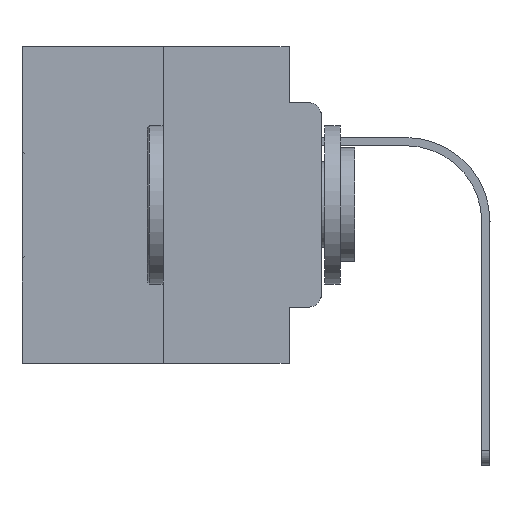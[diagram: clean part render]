
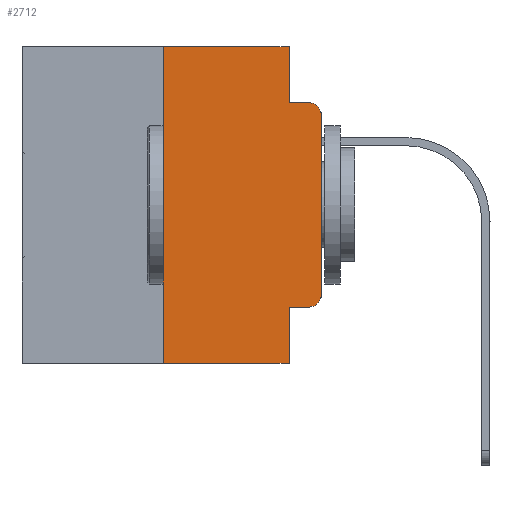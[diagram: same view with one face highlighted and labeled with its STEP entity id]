
A CAD part, left-side view. The second image highlights one B-rep face of the part: STEP entity #2712.
In plain terms, the highlighted planar face has unit normal (-1, 0, 0).
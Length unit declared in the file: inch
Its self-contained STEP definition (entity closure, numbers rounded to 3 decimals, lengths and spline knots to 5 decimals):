
#999 = EDGE_CURVE ( 'NONE', #12765, #30200, #6936, .T. ) ;
#1130 = CARTESIAN_POINT ( 'NONE',  ( 0., 0.25, -0.5 ) ) ;
#1469 = CARTESIAN_POINT ( 'NONE',  ( 0., 0.473, 0. ) ) ;
#1956 = CARTESIAN_POINT ( 'NONE',  ( 0., 0.02, -0.1085 ) ) ;
#2141 = CARTESIAN_POINT ( 'NONE',  ( 0., 0.02, -0.0885 ) ) ;
#2453 = CARTESIAN_POINT ( 'NONE',  ( 0., 0., -0.1085 ) ) ;
#2712 = ADVANCED_FACE ( 'NONE', ( #13245 ), #22692, .F. ) ;
#2751 = CARTESIAN_POINT ( 'NONE',  ( 0., 0.051, 0. ) ) ;
#3183 = ORIENTED_EDGE ( 'NONE', *, *, #10460, .F. ) ;
#3632 = CARTESIAN_POINT ( 'NONE',  ( 0., 0.25, 0. ) ) ;
#3647 = VERTEX_POINT ( 'NONE', #2141 ) ;
#3728 = EDGE_LOOP ( 'NONE', ( #21203, #11281, #12507, #26506, #24095, #4914, #7274, #3183, #17804, #25895 ) ) ;
#3766 = VECTOR ( 'NONE', #8851, 39.37008 ) ;
#4175 = LINE ( 'NONE', #13935, #3766 ) ;
#4287 = DIRECTION ( 'NONE',  ( -1., 0., 0. ) ) ;
#4724 = CARTESIAN_POINT ( 'NONE',  ( 0., 0.051, -0.5 ) ) ;
#4914 = ORIENTED_EDGE ( 'NONE', *, *, #18282, .F. ) ;
#5265 = CARTESIAN_POINT ( 'NONE',  ( 0., 0.051, -0.0885 ) ) ;
#5772 = DIRECTION ( 'NONE',  ( 0., -1., 0. ) ) ;
#6114 = DIRECTION ( 'NONE',  ( 0., 0., -1. ) ) ;
#6195 = AXIS2_PLACEMENT_3D ( 'NONE', #25913, #4287, #29947 ) ;
#6268 = DIRECTION ( 'NONE',  ( 1., 0., 0. ) ) ;
#6936 = LINE ( 'NONE', #25796, #30480 ) ;
#7060 = EDGE_CURVE ( 'NONE', #26510, #7938, #28341, .T. ) ;
#7166 = CARTESIAN_POINT ( 'NONE',  ( 0., 0.473, -0.5 ) ) ;
#7274 = ORIENTED_EDGE ( 'NONE', *, *, #7060, .T. ) ;
#7452 = LINE ( 'NONE', #11924, #13524 ) ;
#7598 = DIRECTION ( 'NONE',  ( 0., 0., 1. ) ) ;
#7938 = VERTEX_POINT ( 'NONE', #4724 ) ;
#8336 = DIRECTION ( 'NONE',  ( 0., -1., 0. ) ) ;
#8405 = CIRCLE ( 'NONE', #12333, 0.02 ) ;
#8851 = DIRECTION ( 'NONE',  ( 0., 0., 1. ) ) ;
#8909 = VERTEX_POINT ( 'NONE', #5265 ) ;
#10203 = VECTOR ( 'NONE', #16624, 39.37008 ) ;
#10460 = EDGE_CURVE ( 'NONE', #18281, #7938, #19195, .T. ) ;
#10653 = CIRCLE ( 'NONE', #6195, 0.02 ) ;
#11222 = VECTOR ( 'NONE', #6114, 39.37008 ) ;
#11281 = ORIENTED_EDGE ( 'NONE', *, *, #26190, .T. ) ;
#11924 = CARTESIAN_POINT ( 'NONE',  ( 0., 0., 0. ) ) ;
#11931 = CARTESIAN_POINT ( 'NONE',  ( 0., 0.051, 0. ) ) ;
#12333 = AXIS2_PLACEMENT_3D ( 'NONE', #1956, #30238, #18697 ) ;
#12507 = ORIENTED_EDGE ( 'NONE', *, *, #17364, .F. ) ;
#12765 = VERTEX_POINT ( 'NONE', #3632 ) ;
#13048 = CARTESIAN_POINT ( 'NONE',  ( 0., 0.051, -0.4115 ) ) ;
#13245 = FACE_OUTER_BOUND ( 'NONE', #3728, .T. ) ;
#13486 = EDGE_CURVE ( 'NONE', #22192, #23273, #7452, .T. ) ;
#13524 = VECTOR ( 'NONE', #7598, 39.37008 ) ;
#13628 = VECTOR ( 'NONE', #8336, 39.37008 ) ;
#13935 = CARTESIAN_POINT ( 'NONE',  ( 0., 0.25, 0. ) ) ;
#13940 = VECTOR ( 'NONE', #27988, 39.37008 ) ;
#15738 = DIRECTION ( 'NONE',  ( 0., 0., -1. ) ) ;
#16624 = DIRECTION ( 'NONE',  ( 0., -1., 0. ) ) ;
#17326 = CARTESIAN_POINT ( 'NONE',  ( 0., 0.051, -0.0885 ) ) ;
#17364 = EDGE_CURVE ( 'NONE', #8909, #3647, #24421, .T. ) ;
#17754 = LINE ( 'NONE', #29457, #11222 ) ;
#17804 = ORIENTED_EDGE ( 'NONE', *, *, #29872, .T. ) ;
#18281 = VERTEX_POINT ( 'NONE', #30154 ) ;
#18282 = EDGE_CURVE ( 'NONE', #26510, #12765, #4175, .T. ) ;
#18697 = DIRECTION ( 'NONE',  ( 0., 0., -1. ) ) ;
#19195 = LINE ( 'NONE', #2751, #13940 ) ;
#21183 = CARTESIAN_POINT ( 'NONE',  ( 0., 0.02, -0.4115 ) ) ;
#21203 = ORIENTED_EDGE ( 'NONE', *, *, #13486, .T. ) ;
#22192 = VERTEX_POINT ( 'NONE', #28868 ) ;
#22471 = VERTEX_POINT ( 'NONE', #21183 ) ;
#22692 = PLANE ( 'NONE',  #29877 ) ;
#23273 = VERTEX_POINT ( 'NONE', #2453 ) ;
#24092 = VECTOR ( 'NONE', #5772, 39.37008 ) ;
#24095 = ORIENTED_EDGE ( 'NONE', *, *, #999, .F. ) ;
#24421 = LINE ( 'NONE', #17326, #13628 ) ;
#25796 = CARTESIAN_POINT ( 'NONE',  ( 0., 0.473, 0. ) ) ;
#25895 = ORIENTED_EDGE ( 'NONE', *, *, #27807, .T. ) ;
#25913 = CARTESIAN_POINT ( 'NONE',  ( 0., 0.02, -0.3915 ) ) ;
#26190 = EDGE_CURVE ( 'NONE', #23273, #3647, #8405, .T. ) ;
#26506 = ORIENTED_EDGE ( 'NONE', *, *, #29414, .F. ) ;
#26510 = VERTEX_POINT ( 'NONE', #1130 ) ;
#27121 = LINE ( 'NONE', #13048, #24092 ) ;
#27807 = EDGE_CURVE ( 'NONE', #22471, #22192, #10653, .T. ) ;
#27988 = DIRECTION ( 'NONE',  ( 0., 0., -1. ) ) ;
#28341 = LINE ( 'NONE', #7166, #10203 ) ;
#28868 = CARTESIAN_POINT ( 'NONE',  ( 0., 0., -0.3915 ) ) ;
#29414 = EDGE_CURVE ( 'NONE', #30200, #8909, #17754, .T. ) ;
#29457 = CARTESIAN_POINT ( 'NONE',  ( 0., 0.051, 0. ) ) ;
#29872 = EDGE_CURVE ( 'NONE', #18281, #22471, #27121, .T. ) ;
#29877 = AXIS2_PLACEMENT_3D ( 'NONE', #1469, #6268, #15738 ) ;
#29947 = DIRECTION ( 'NONE',  ( 0., 0., -1. ) ) ;
#30154 = CARTESIAN_POINT ( 'NONE',  ( 0., 0.051, -0.4115 ) ) ;
#30200 = VERTEX_POINT ( 'NONE', #11931 ) ;
#30238 = DIRECTION ( 'NONE',  ( -1., 0., 0. ) ) ;
#30272 = DIRECTION ( 'NONE',  ( 0., -1., 0. ) ) ;
#30480 = VECTOR ( 'NONE', #30272, 39.37008 ) ;
